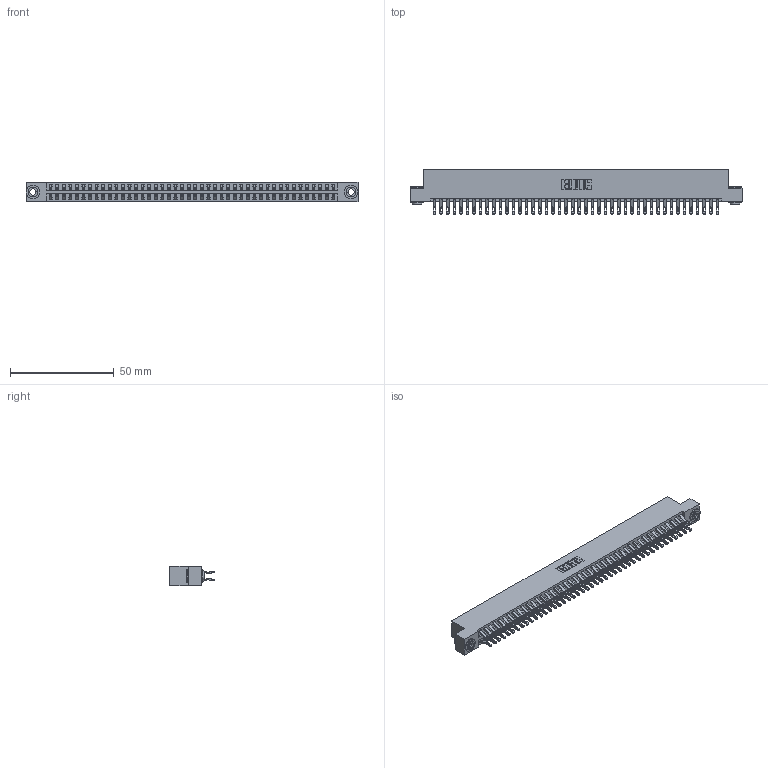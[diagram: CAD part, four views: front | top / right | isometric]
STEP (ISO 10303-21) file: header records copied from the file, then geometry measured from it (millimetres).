
FILE_DESCRIPTION (( 'STEP AP203' ), '1' );
FILE_NAME ('396-088-555-203.STEP', '2018-09-10T06:22:01', ( '' ), ( '' ), 'SwSTEP 2.0', 'SolidWorks 2016', '' );
FILE_SCHEMA (( 'CONFIG_CONTROL_DESIGN' ));
Length unit declared in the file: inch
Products named in the file (4): 345-292-001_555 Tail; 345-250-002_345-250-002-102; 396-088-555-203; 346 Part_Flush Mounting Lugs - 0.156 Dia-TH
Assembly tree (91 placements, depth 2):
  396-088-555-203
    346 Part_Flush Mounting Lugs - 0.156 Dia-TH
    345-292-001_555 Tail  x88
    345-250-002_345-250-002-102  x2
Bounding box: 160.27 x 21.46 x 9.4 mm (x, y, z)
Volume: 15918.9 mm3; surface area: 23037.1 mm2
Topology: 91 solids, 91 shells, 5264 faces, 16509 edges, 11002 vertices
Faces by surface type: plane 2990, cylinder 2266, cone 8
Entity records: 29422 total; most frequent: CARTESIAN_POINT 4857, ORIENTED_EDGE 4754, DIRECTION 4331, EDGE_CURVE 2377, VECTOR 2025, LINE 2025, VERTEX_POINT 1582, AXIS2_PLACEMENT_3D 1153
